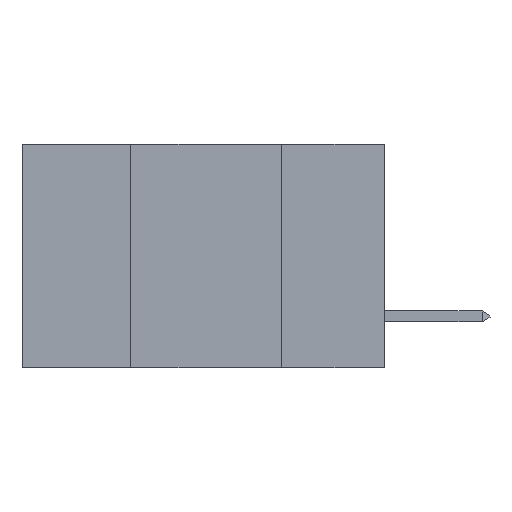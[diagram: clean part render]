
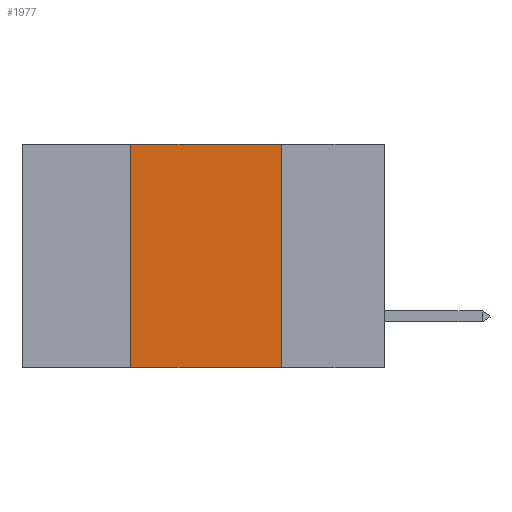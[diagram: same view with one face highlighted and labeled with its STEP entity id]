
A CAD part, left-side view. The second image highlights one B-rep face of the part: STEP entity #1977.
In plain terms, the highlighted planar face has unit normal (-1, 0, 0).
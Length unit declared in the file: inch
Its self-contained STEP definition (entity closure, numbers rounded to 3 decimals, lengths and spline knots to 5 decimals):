
#49 = VERTEX_POINT ( 'NONE', #3604 ) ;
#733 = VECTOR ( 'NONE', #2615, 39.37008 ) ;
#879 = LINE ( 'NONE', #8523, #5673 ) ;
#1681 = VERTEX_POINT ( 'NONE', #8278 ) ;
#1977 = ADVANCED_FACE ( 'NONE', ( #12078 ), #7123, .F. ) ;
#2112 = CARTESIAN_POINT ( 'NONE',  ( 0., 0.17, -0.37 ) ) ;
#2615 = DIRECTION ( 'NONE',  ( 0., -1., 0. ) ) ;
#2808 = DIRECTION ( 'NONE',  ( 0., -1., 0. ) ) ;
#3362 = LINE ( 'NONE', #9033, #733 ) ;
#3604 = CARTESIAN_POINT ( 'NONE',  ( 0., 0.42, -0.37 ) ) ;
#3806 = EDGE_CURVE ( 'NONE', #49, #1681, #3984, .T. ) ;
#3984 = LINE ( 'NONE', #6694, #10979 ) ;
#5673 = VECTOR ( 'NONE', #7655, 39.37008 ) ;
#5957 = CARTESIAN_POINT ( 'NONE',  ( 0., 0.6, 0. ) ) ;
#6398 = VECTOR ( 'NONE', #2808, 39.37008 ) ;
#6651 = EDGE_CURVE ( 'NONE', #7885, #8234, #879, .T. ) ;
#6694 = CARTESIAN_POINT ( 'NONE',  ( 0., 0.42, 0. ) ) ;
#6793 = DIRECTION ( 'NONE',  ( 0., 0., 1. ) ) ;
#6799 = DIRECTION ( 'NONE',  ( 1., 0., 0. ) ) ;
#7008 = ORIENTED_EDGE ( 'NONE', *, *, #10773, .T. ) ;
#7123 = PLANE ( 'NONE',  #9503 ) ;
#7346 = CARTESIAN_POINT ( 'NONE',  ( 0., 0.17, 0. ) ) ;
#7655 = DIRECTION ( 'NONE',  ( 0., 0., -1. ) ) ;
#7885 = VERTEX_POINT ( 'NONE', #7346 ) ;
#8234 = VERTEX_POINT ( 'NONE', #2112 ) ;
#8278 = CARTESIAN_POINT ( 'NONE',  ( 0., 0.42, 0. ) ) ;
#8297 = CARTESIAN_POINT ( 'NONE',  ( 0., 0.6, 0. ) ) ;
#8356 = EDGE_LOOP ( 'NONE', ( #10037, #9253, #9572, #7008 ) ) ;
#8523 = CARTESIAN_POINT ( 'NONE',  ( 0., 0.17, 0. ) ) ;
#9033 = CARTESIAN_POINT ( 'NONE',  ( 0., 0.6, -0.37 ) ) ;
#9253 = ORIENTED_EDGE ( 'NONE', *, *, #9496, .F. ) ;
#9496 = EDGE_CURVE ( 'NONE', #1681, #7885, #11228, .T. ) ;
#9503 = AXIS2_PLACEMENT_3D ( 'NONE', #5957, #6799, #11833 ) ;
#9572 = ORIENTED_EDGE ( 'NONE', *, *, #3806, .F. ) ;
#10037 = ORIENTED_EDGE ( 'NONE', *, *, #6651, .F. ) ;
#10773 = EDGE_CURVE ( 'NONE', #49, #8234, #3362, .T. ) ;
#10979 = VECTOR ( 'NONE', #6793, 39.37008 ) ;
#11228 = LINE ( 'NONE', #8297, #6398 ) ;
#11833 = DIRECTION ( 'NONE',  ( 0., 0., -1. ) ) ;
#12078 = FACE_OUTER_BOUND ( 'NONE', #8356, .T. ) ;
